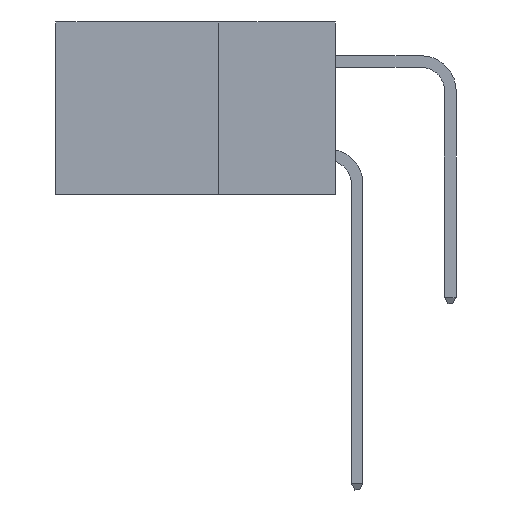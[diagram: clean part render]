
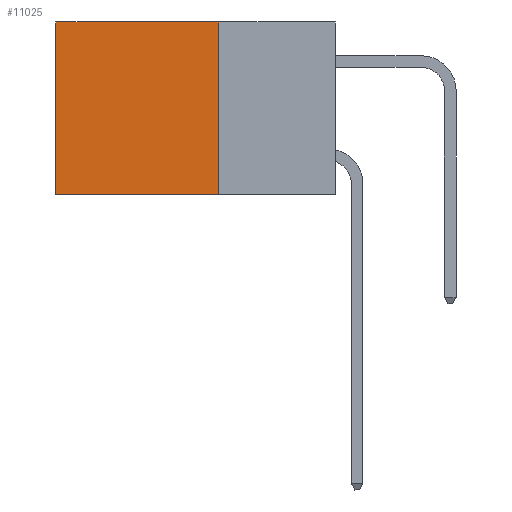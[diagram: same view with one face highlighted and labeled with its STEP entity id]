
A CAD part, left-side view. The second image highlights one B-rep face of the part: STEP entity #11025.
In plain terms, the highlighted planar face has unit normal (-1, 0, 0).
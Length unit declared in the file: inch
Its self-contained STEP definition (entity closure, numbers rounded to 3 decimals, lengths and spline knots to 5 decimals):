
#524 = VERTEX_POINT ( 'NONE', #11294 ) ;
#596 = CARTESIAN_POINT ( 'NONE',  ( 0.2875, 0.6, 0. ) ) ;
#882 = VECTOR ( 'NONE', #13966, 39.37008 ) ;
#1218 = DIRECTION ( 'NONE',  ( 0., 0., -1. ) ) ;
#1341 = LINE ( 'NONE', #12579, #882 ) ;
#1620 = ORIENTED_EDGE ( 'NONE', *, *, #16889, .T. ) ;
#2706 = LINE ( 'NONE', #9869, #17714 ) ;
#3545 = VERTEX_POINT ( 'NONE', #10119 ) ;
#4439 = ORIENTED_EDGE ( 'NONE', *, *, #10552, .F. ) ;
#4750 = LINE ( 'NONE', #14438, #8111 ) ;
#6548 = EDGE_LOOP ( 'NONE', ( #1620, #16898, #4439, #10567 ) ) ;
#6916 = EDGE_CURVE ( 'NONE', #524, #3545, #4750, .T. ) ;
#7574 = AXIS2_PLACEMENT_3D ( 'NONE', #7982, #17789, #9465 ) ;
#7982 = CARTESIAN_POINT ( 'NONE',  ( 0.2875, 0.25, 0. ) ) ;
#8111 = VECTOR ( 'NONE', #14373, 39.37008 ) ;
#8243 = VERTEX_POINT ( 'NONE', #14960 ) ;
#8580 = VECTOR ( 'NONE', #13613, 39.37008 ) ;
#9048 = LINE ( 'NONE', #12217, #8580 ) ;
#9465 = DIRECTION ( 'NONE',  ( 0., 0., -1. ) ) ;
#9595 = VERTEX_POINT ( 'NONE', #596 ) ;
#9869 = CARTESIAN_POINT ( 'NONE',  ( 0.2875, 0.25, 0. ) ) ;
#10119 = CARTESIAN_POINT ( 'NONE',  ( 0.2875, 0.6, -0.37 ) ) ;
#10326 = FACE_OUTER_BOUND ( 'NONE', #6548, .T. ) ;
#10552 = EDGE_CURVE ( 'NONE', #8243, #524, #2706, .T. ) ;
#10567 = ORIENTED_EDGE ( 'NONE', *, *, #14997, .T. ) ;
#11025 = ADVANCED_FACE ( 'NONE', ( #10326 ), #16394, .F. ) ;
#11294 = CARTESIAN_POINT ( 'NONE',  ( 0.2875, 0.25, -0.37 ) ) ;
#12217 = CARTESIAN_POINT ( 'NONE',  ( 0.2875, 0.25, 0. ) ) ;
#12579 = CARTESIAN_POINT ( 'NONE',  ( 0.2875, 0.6, 0. ) ) ;
#13613 = DIRECTION ( 'NONE',  ( 0., 1., 0. ) ) ;
#13966 = DIRECTION ( 'NONE',  ( 0., 0., -1. ) ) ;
#14373 = DIRECTION ( 'NONE',  ( 0., 1., 0. ) ) ;
#14438 = CARTESIAN_POINT ( 'NONE',  ( 0.2875, 0.25, -0.37 ) ) ;
#14960 = CARTESIAN_POINT ( 'NONE',  ( 0.2875, 0.25, 0. ) ) ;
#14997 = EDGE_CURVE ( 'NONE', #8243, #9595, #9048, .T. ) ;
#16394 = PLANE ( 'NONE',  #7574 ) ;
#16889 = EDGE_CURVE ( 'NONE', #9595, #3545, #1341, .T. ) ;
#16898 = ORIENTED_EDGE ( 'NONE', *, *, #6916, .F. ) ;
#17714 = VECTOR ( 'NONE', #1218, 39.37008 ) ;
#17789 = DIRECTION ( 'NONE',  ( 1., 0., 0. ) ) ;
